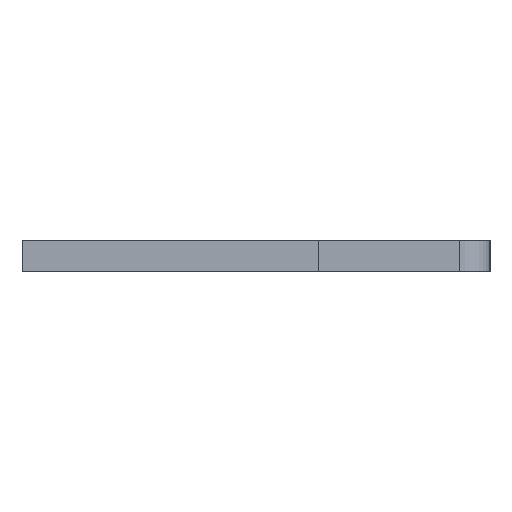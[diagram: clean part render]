
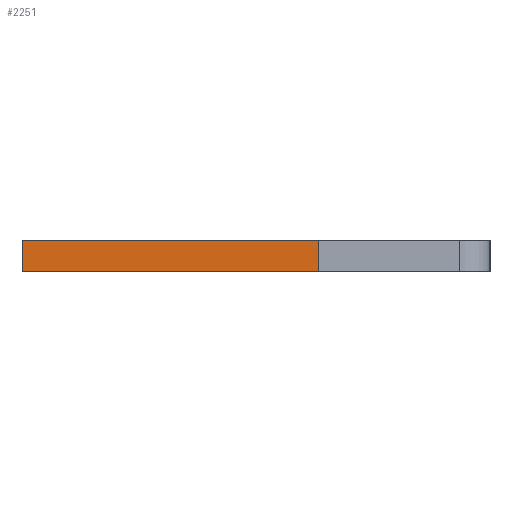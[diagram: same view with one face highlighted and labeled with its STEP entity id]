
A CAD part, left-side view. The second image highlights one B-rep face of the part: STEP entity #2251.
In plain terms, the highlighted face is planar.
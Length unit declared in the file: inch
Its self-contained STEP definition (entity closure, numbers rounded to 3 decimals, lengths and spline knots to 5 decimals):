
#16 = EDGE_CURVE ( 'NONE', #2338, #448, #2200, .T. ) ;
#290 = ORIENTED_EDGE ( 'NONE', *, *, #2689, .T. ) ;
#352 = LINE ( 'NONE', #2732, #430 ) ;
#366 = CARTESIAN_POINT ( 'NONE',  ( -0.01, -0.04, -0.04 ) ) ;
#430 = VECTOR ( 'NONE', #2243, 39.37008 ) ;
#448 = VERTEX_POINT ( 'NONE', #1579 ) ;
#779 = DIRECTION ( 'NONE',  ( -1., 0., 0. ) ) ;
#901 = DIRECTION ( 'NONE',  ( 0., 0., 1. ) ) ;
#1007 = EDGE_CURVE ( 'NONE', #2465, #2514, #1416, .T. ) ;
#1173 = VECTOR ( 'NONE', #2905, 39.37008 ) ;
#1335 = FACE_OUTER_BOUND ( 'NONE', #2073, .T. ) ;
#1386 = ORIENTED_EDGE ( 'NONE', *, *, #1007, .T. ) ;
#1416 = LINE ( 'NONE', #2892, #2236 ) ;
#1579 = CARTESIAN_POINT ( 'NONE',  ( -0.01, 0.15, -0.04 ) ) ;
#1623 = CARTESIAN_POINT ( 'NONE',  ( 0.01, 0.15, -0.04 ) ) ;
#1633 = CARTESIAN_POINT ( 'NONE',  ( 0.01, 0.15, -0.04 ) ) ;
#1668 = AXIS2_PLACEMENT_3D ( 'NONE', #1633, #901, #2399 ) ;
#1909 = PLANE ( 'NONE',  #1668 ) ;
#2011 = CARTESIAN_POINT ( 'NONE',  ( 0.01, 0.15, -0.04 ) ) ;
#2073 = EDGE_LOOP ( 'NONE', ( #290, #2210, #2763, #1386 ) ) ;
#2143 = DIRECTION ( 'NONE',  ( -1., 0., 0. ) ) ;
#2145 = CARTESIAN_POINT ( 'NONE',  ( 0.01, -0.04, -0.04 ) ) ;
#2200 = LINE ( 'NONE', #2011, #2962 ) ;
#2210 = ORIENTED_EDGE ( 'NONE', *, *, #16, .F. ) ;
#2236 = VECTOR ( 'NONE', #2143, 39.37008 ) ;
#2243 = DIRECTION ( 'NONE',  ( 0., 1., 0. ) ) ;
#2251 = ADVANCED_FACE ( 'NONE', ( #1335 ), #1909, .F. ) ;
#2338 = VERTEX_POINT ( 'NONE', #1623 ) ;
#2383 = CARTESIAN_POINT ( 'NONE',  ( -0.01, 0.15, -0.04 ) ) ;
#2399 = DIRECTION ( 'NONE',  ( 1., 0., 0. ) ) ;
#2465 = VERTEX_POINT ( 'NONE', #2145 ) ;
#2514 = VERTEX_POINT ( 'NONE', #366 ) ;
#2689 = EDGE_CURVE ( 'NONE', #2514, #448, #3110, .T. ) ;
#2732 = CARTESIAN_POINT ( 'NONE',  ( 0.01, 0.15, -0.04 ) ) ;
#2763 = ORIENTED_EDGE ( 'NONE', *, *, #3108, .F. ) ;
#2892 = CARTESIAN_POINT ( 'NONE',  ( 0.01, -0.04, -0.04 ) ) ;
#2905 = DIRECTION ( 'NONE',  ( 0., 1., 0. ) ) ;
#2962 = VECTOR ( 'NONE', #779, 39.37008 ) ;
#3108 = EDGE_CURVE ( 'NONE', #2465, #2338, #352, .T. ) ;
#3110 = LINE ( 'NONE', #2383, #1173 ) ;
